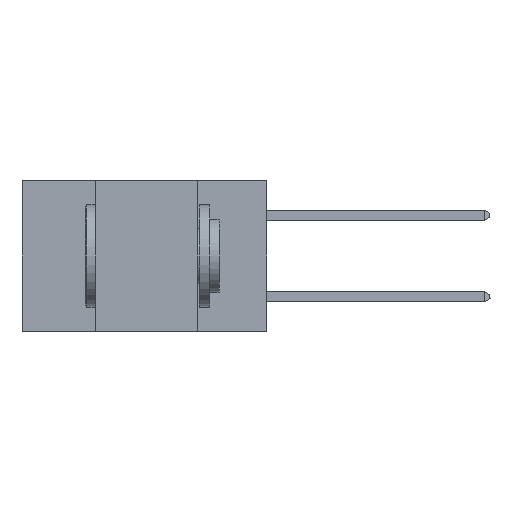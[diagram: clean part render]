
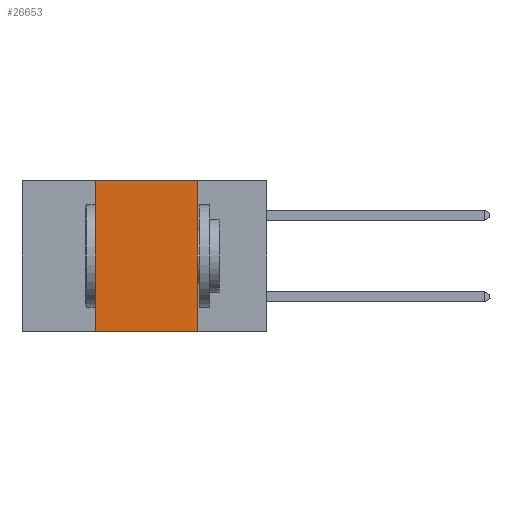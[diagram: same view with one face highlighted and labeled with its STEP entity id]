
A CAD part, left-side view. The second image highlights one B-rep face of the part: STEP entity #26653.
In plain terms, the highlighted planar face has unit normal (-1, 0, 0).
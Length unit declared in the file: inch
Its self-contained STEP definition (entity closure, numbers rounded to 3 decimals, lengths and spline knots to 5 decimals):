
#158 = VECTOR ( 'NONE', #25343, 39.37008 ) ;
#2235 = ORIENTED_EDGE ( 'NONE', *, *, #22878, .F. ) ;
#4466 = DIRECTION ( 'NONE',  ( 0., 0., -1. ) ) ;
#5164 = CARTESIAN_POINT ( 'NONE',  ( 0., 0.42, 0. ) ) ;
#5196 = CARTESIAN_POINT ( 'NONE',  ( 0., 0.6, -0.37 ) ) ;
#5367 = DIRECTION ( 'NONE',  ( 0., 0., 1. ) ) ;
#7978 = DIRECTION ( 'NONE',  ( 0., -1., 0. ) ) ;
#8608 = LINE ( 'NONE', #15907, #158 ) ;
#8611 = CARTESIAN_POINT ( 'NONE',  ( 0., 0.17, -0.37 ) ) ;
#10228 = EDGE_CURVE ( 'NONE', #16929, #15370, #8608, .T. ) ;
#10286 = EDGE_CURVE ( 'NONE', #28087, #16929, #26325, .T. ) ;
#10842 = AXIS2_PLACEMENT_3D ( 'NONE', #15986, #16073, #4466 ) ;
#10877 = EDGE_CURVE ( 'NONE', #28804, #15370, #11497, .T. ) ;
#11497 = LINE ( 'NONE', #5196, #12970 ) ;
#12807 = ORIENTED_EDGE ( 'NONE', *, *, #10286, .F. ) ;
#12970 = VECTOR ( 'NONE', #21671, 39.37008 ) ;
#14272 = CARTESIAN_POINT ( 'NONE',  ( 0., 0.42, 0. ) ) ;
#15203 = VECTOR ( 'NONE', #7978, 39.37008 ) ;
#15370 = VERTEX_POINT ( 'NONE', #8611 ) ;
#15907 = CARTESIAN_POINT ( 'NONE',  ( 0., 0.17, 0. ) ) ;
#15986 = CARTESIAN_POINT ( 'NONE',  ( 0., 0.6, 0. ) ) ;
#16071 = CARTESIAN_POINT ( 'NONE',  ( 0., 0.42, -0.37 ) ) ;
#16073 = DIRECTION ( 'NONE',  ( 1., 0., 0. ) ) ;
#16929 = VERTEX_POINT ( 'NONE', #30093 ) ;
#17858 = CARTESIAN_POINT ( 'NONE',  ( 0., 0.6, 0. ) ) ;
#21671 = DIRECTION ( 'NONE',  ( 0., -1., 0. ) ) ;
#22878 = EDGE_CURVE ( 'NONE', #28804, #28087, #30460, .T. ) ;
#25338 = EDGE_LOOP ( 'NONE', ( #27649, #12807, #2235, #29009 ) ) ;
#25343 = DIRECTION ( 'NONE',  ( 0., 0., -1. ) ) ;
#25758 = FACE_OUTER_BOUND ( 'NONE', #25338, .T. ) ;
#26325 = LINE ( 'NONE', #17858, #15203 ) ;
#26653 = ADVANCED_FACE ( 'NONE', ( #25758 ), #27973, .F. ) ;
#27649 = ORIENTED_EDGE ( 'NONE', *, *, #10228, .F. ) ;
#27973 = PLANE ( 'NONE',  #10842 ) ;
#28087 = VERTEX_POINT ( 'NONE', #14272 ) ;
#28231 = VECTOR ( 'NONE', #5367, 39.37008 ) ;
#28804 = VERTEX_POINT ( 'NONE', #16071 ) ;
#29009 = ORIENTED_EDGE ( 'NONE', *, *, #10877, .T. ) ;
#30093 = CARTESIAN_POINT ( 'NONE',  ( 0., 0.17, 0. ) ) ;
#30460 = LINE ( 'NONE', #5164, #28231 ) ;
